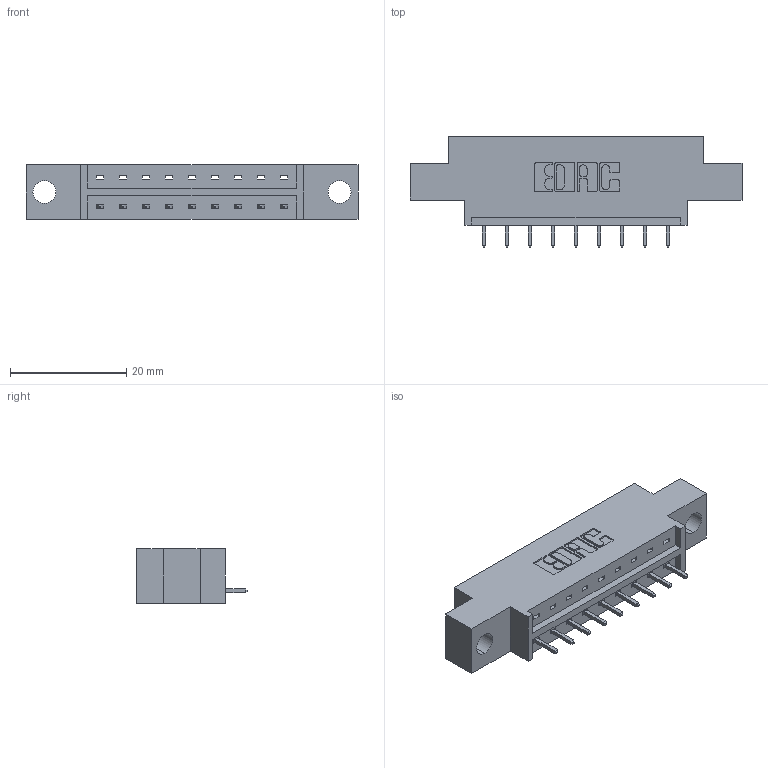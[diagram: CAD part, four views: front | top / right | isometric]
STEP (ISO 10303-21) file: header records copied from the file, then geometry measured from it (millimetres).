
FILE_DESCRIPTION (( 'STEP AP203' ), '1' );
FILE_NAME ('833-009-521-604.STEP', '2020-05-30T17:02:04', ( '' ), ( '' ), 'SwSTEP 2.0', 'SolidWorks 2020', '' );
FILE_SCHEMA (( 'CONFIG_CONTROL_DESIGN' ));
Length unit declared in the file: inch
Products named in the file (3): 833 Part_Offset - .156 Dia - TH; 833-009-521-604; 345-292-001_345-293-121
Assembly tree (10 placements, depth 2):
  833-009-521-604
    833 Part_Offset - .156 Dia - TH
    345-292-001_345-293-121  x9
Bounding box: 57.2 x 19.06 x 9.4 mm (x, y, z)
Volume: 5131 mm3; surface area: 5222.7 mm2
Topology: 10 solids, 10 shells, 640 faces, 1907 edges, 1258 vertices
Faces by surface type: plane 452, cylinder 188
Entity records: 9923 total; most frequent: CARTESIAN_POINT 1725, ORIENTED_EDGE 1670, DIRECTION 1521, EDGE_CURVE 835, LINE 707, VECTOR 707, VERTEX_POINT 554, AXIS2_PLACEMENT_3D 407
